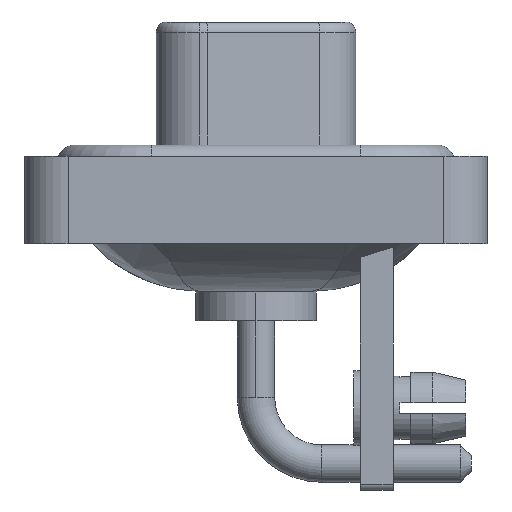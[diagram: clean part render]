
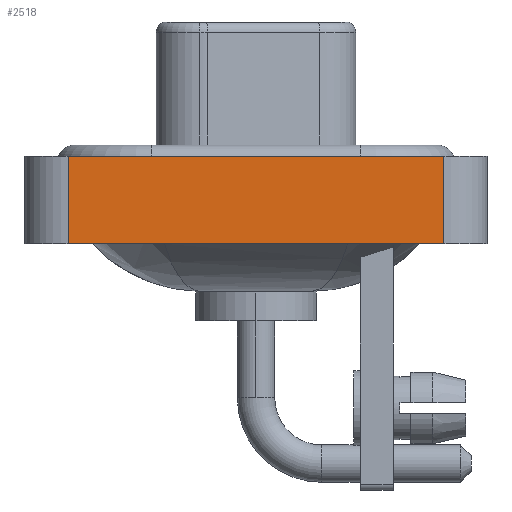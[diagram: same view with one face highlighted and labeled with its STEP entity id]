
A CAD part, left-side view. The second image highlights one B-rep face of the part: STEP entity #2518.
In plain terms, the highlighted planar face has unit normal (-1, 0, 0).
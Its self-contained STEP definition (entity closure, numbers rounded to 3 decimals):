
#130 = DIRECTION ( 'NONE',  ( 0., 0., 1. ) ) ;
#232 = CARTESIAN_POINT ( 'NONE',  ( -7.25, -8.55, -3.6 ) ) ;
#292 = DIRECTION ( 'NONE',  ( 0., -1., 0. ) ) ;
#309 = CARTESIAN_POINT ( 'NONE',  ( -7.25, 8.55, -3.6 ) ) ;
#313 = VERTEX_POINT ( 'NONE', #309 ) ;
#914 = CARTESIAN_POINT ( 'NONE',  ( -7.25, 8.55, 0.4 ) ) ;
#1208 = EDGE_CURVE ( 'NONE', #6642, #16034, #5690, .T. ) ;
#2518 = ADVANCED_FACE ( 'NONE', ( #16227 ), #12154, .T. ) ;
#2616 = DIRECTION ( 'NONE',  ( 0., -1., 0. ) ) ;
#2874 = VECTOR ( 'NONE', #130, 1000. ) ;
#3028 = ORIENTED_EDGE ( 'NONE', *, *, #9972, .T. ) ;
#3627 = VECTOR ( 'NONE', #8432, 1000. ) ;
#4206 = CARTESIAN_POINT ( 'NONE',  ( -7.25, -8.55, -3.6 ) ) ;
#4282 = DIRECTION ( 'NONE',  ( 0., 0., 1. ) ) ;
#4311 = EDGE_CURVE ( 'NONE', #313, #7211, #6838, .T. ) ;
#4623 = CARTESIAN_POINT ( 'NONE',  ( -7.25, -8.55, 0.4 ) ) ;
#5274 = LINE ( 'NONE', #232, #17050 ) ;
#5443 = DIRECTION ( 'NONE',  ( -1., 0., 0. ) ) ;
#5676 = LINE ( 'NONE', #4623, #16359 ) ;
#5690 = LINE ( 'NONE', #5781, #3627 ) ;
#5781 = CARTESIAN_POINT ( 'NONE',  ( -7.25, -8.55, -3.6 ) ) ;
#6642 = VERTEX_POINT ( 'NONE', #16502 ) ;
#6838 = LINE ( 'NONE', #12238, #2874 ) ;
#7211 = VERTEX_POINT ( 'NONE', #914 ) ;
#7545 = EDGE_CURVE ( 'NONE', #7211, #16034, #5676, .T. ) ;
#7574 = AXIS2_PLACEMENT_3D ( 'NONE', #4206, #5443, #4282 ) ;
#8397 = ORIENTED_EDGE ( 'NONE', *, *, #4311, .F. ) ;
#8432 = DIRECTION ( 'NONE',  ( 0., 0., 1. ) ) ;
#9972 = EDGE_CURVE ( 'NONE', #313, #6642, #5274, .T. ) ;
#10085 = ORIENTED_EDGE ( 'NONE', *, *, #1208, .T. ) ;
#10720 = ORIENTED_EDGE ( 'NONE', *, *, #7545, .F. ) ;
#12154 = PLANE ( 'NONE',  #7574 ) ;
#12238 = CARTESIAN_POINT ( 'NONE',  ( -7.25, 8.55, -3.6 ) ) ;
#12733 = EDGE_LOOP ( 'NONE', ( #10085, #10720, #8397, #3028 ) ) ;
#13779 = CARTESIAN_POINT ( 'NONE',  ( -7.25, -8.55, 0.4 ) ) ;
#16034 = VERTEX_POINT ( 'NONE', #13779 ) ;
#16227 = FACE_OUTER_BOUND ( 'NONE', #12733, .T. ) ;
#16359 = VECTOR ( 'NONE', #292, 1000. ) ;
#16502 = CARTESIAN_POINT ( 'NONE',  ( -7.25, -8.55, -3.6 ) ) ;
#17050 = VECTOR ( 'NONE', #2616, 1000. ) ;
